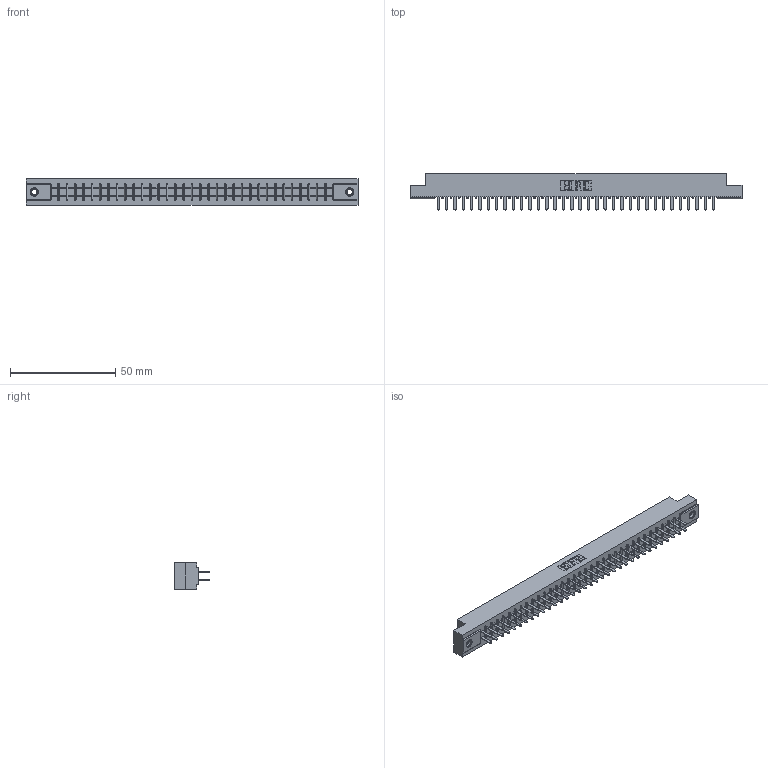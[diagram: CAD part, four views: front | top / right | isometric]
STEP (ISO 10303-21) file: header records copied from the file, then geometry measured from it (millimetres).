
FILE_DESCRIPTION (( 'STEP AP203' ), '1' );
FILE_NAME ('355-068-520-507.STEP', '2019-09-12T16:53:58', ( '' ), ( '' ), 'SwSTEP 2.0', 'SolidWorks 2016', '' );
FILE_SCHEMA (( 'CONFIG_CONTROL_DESIGN' ));
Length unit declared in the file: inch
Products named in the file (4): 305-290-001_520; 355-068-520-507; 345-250-001_345-250-005-103; 305 Part_.156 Dia
Assembly tree (71 placements, depth 2):
  355-068-520-507
    305 Part_.156 Dia
    305-290-001_520  x68
    345-250-001_345-250-005-103  x2
Bounding box: 157.73 x 17.09 x 12.7 mm (x, y, z)
Volume: 15917.6 mm3; surface area: 20907.8 mm2
Topology: 71 solids, 71 shells, 3304 faces, 9394 edges, 6072 vertices
Faces by surface type: plane 1936, cylinder 1216, sphere 136, cone 12, torus 4
Entity records: 38852 total; most frequent: CARTESIAN_POINT 6411, ORIENTED_EDGE 6356, DIRECTION 6218, EDGE_CURVE 3178, LINE 2560, VECTOR 2560, VERTEX_POINT 2022, AXIS2_PLACEMENT_3D 1829
